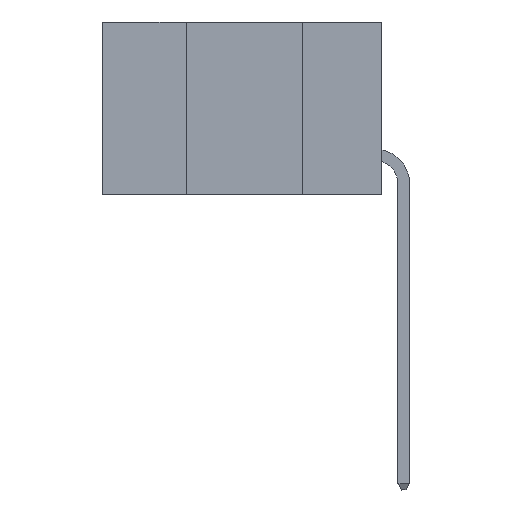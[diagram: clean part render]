
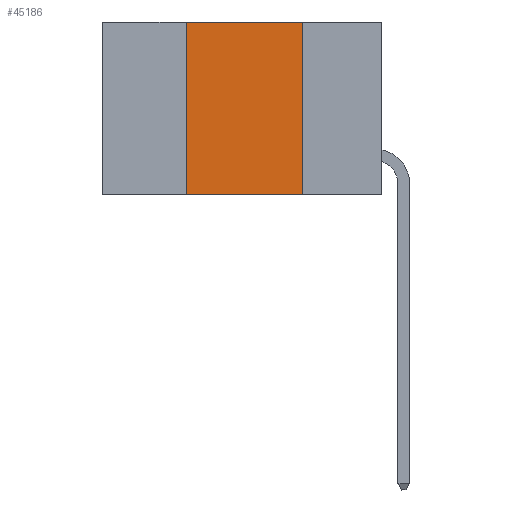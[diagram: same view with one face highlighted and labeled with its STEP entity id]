
A CAD part, left-side view. The second image highlights one B-rep face of the part: STEP entity #45186.
In plain terms, the highlighted planar face has unit normal (-1, 0, 0).
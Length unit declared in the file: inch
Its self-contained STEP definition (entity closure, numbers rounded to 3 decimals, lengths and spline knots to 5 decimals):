
#161 = EDGE_CURVE ( 'NONE', #30713, #45302, #8861, .T. ) ;
#1439 = VECTOR ( 'NONE', #46783, 39.37008 ) ;
#2560 = CARTESIAN_POINT ( 'NONE',  ( 0., 0.17, 0. ) ) ;
#4554 = LINE ( 'NONE', #25903, #1439 ) ;
#4685 = LINE ( 'NONE', #29638, #12520 ) ;
#6008 = CARTESIAN_POINT ( 'NONE',  ( 0., 0.6, 0. ) ) ;
#6009 = AXIS2_PLACEMENT_3D ( 'NONE', #6008, #25586, #32882 ) ;
#6795 = DIRECTION ( 'NONE',  ( 0., 0., 1. ) ) ;
#8033 = VERTEX_POINT ( 'NONE', #2560 ) ;
#8861 = LINE ( 'NONE', #22973, #42501 ) ;
#12520 = VECTOR ( 'NONE', #21603, 39.37008 ) ;
#12746 = DIRECTION ( 'NONE',  ( 0., -1., 0. ) ) ;
#15360 = VECTOR ( 'NONE', #12746, 39.37008 ) ;
#17526 = CARTESIAN_POINT ( 'NONE',  ( 0., 0.42, -0.37 ) ) ;
#17541 = EDGE_CURVE ( 'NONE', #45302, #8033, #47526, .T. ) ;
#17775 = ORIENTED_EDGE ( 'NONE', *, *, #161, .F. ) ;
#20051 = ORIENTED_EDGE ( 'NONE', *, *, #25630, .F. ) ;
#21517 = ORIENTED_EDGE ( 'NONE', *, *, #47441, .T. ) ;
#21603 = DIRECTION ( 'NONE',  ( 0., -1., 0. ) ) ;
#22973 = CARTESIAN_POINT ( 'NONE',  ( 0., 0.42, 0. ) ) ;
#23353 = FACE_OUTER_BOUND ( 'NONE', #46639, .T. ) ;
#25586 = DIRECTION ( 'NONE',  ( 1., 0., 0. ) ) ;
#25630 = EDGE_CURVE ( 'NONE', #8033, #31996, #4554, .T. ) ;
#25903 = CARTESIAN_POINT ( 'NONE',  ( 0., 0.17, 0. ) ) ;
#28285 = PLANE ( 'NONE',  #6009 ) ;
#29638 = CARTESIAN_POINT ( 'NONE',  ( 0., 0.6, -0.37 ) ) ;
#30713 = VERTEX_POINT ( 'NONE', #17526 ) ;
#31996 = VERTEX_POINT ( 'NONE', #47257 ) ;
#32545 = CARTESIAN_POINT ( 'NONE',  ( 0., 0.6, 0. ) ) ;
#32882 = DIRECTION ( 'NONE',  ( 0., 0., -1. ) ) ;
#42501 = VECTOR ( 'NONE', #6795, 39.37008 ) ;
#45186 = ADVANCED_FACE ( 'NONE', ( #23353 ), #28285, .F. ) ;
#45302 = VERTEX_POINT ( 'NONE', #46411 ) ;
#46411 = CARTESIAN_POINT ( 'NONE',  ( 0., 0.42, 0. ) ) ;
#46639 = EDGE_LOOP ( 'NONE', ( #20051, #49268, #17775, #21517 ) ) ;
#46783 = DIRECTION ( 'NONE',  ( 0., 0., -1. ) ) ;
#47257 = CARTESIAN_POINT ( 'NONE',  ( 0., 0.17, -0.37 ) ) ;
#47441 = EDGE_CURVE ( 'NONE', #30713, #31996, #4685, .T. ) ;
#47526 = LINE ( 'NONE', #32545, #15360 ) ;
#49268 = ORIENTED_EDGE ( 'NONE', *, *, #17541, .F. ) ;
